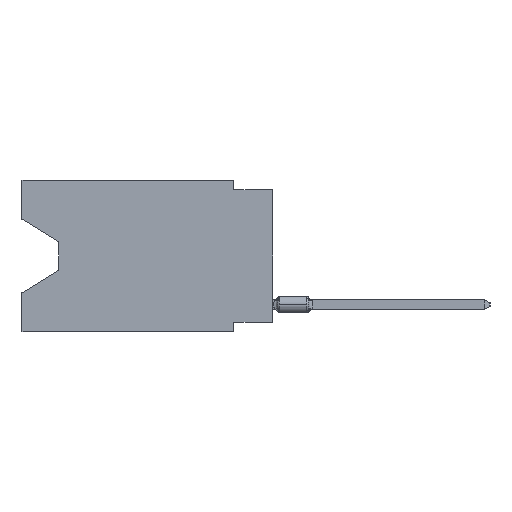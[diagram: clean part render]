
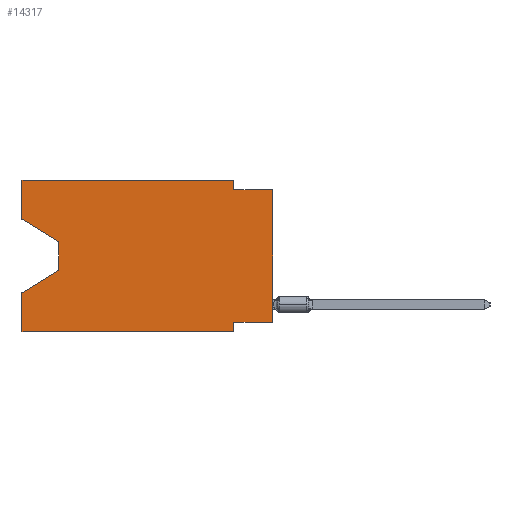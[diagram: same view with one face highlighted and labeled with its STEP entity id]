
A CAD part, left-side view. The second image highlights one B-rep face of the part: STEP entity #14317.
In plain terms, the highlighted planar face has unit normal (-1, 0, 0).
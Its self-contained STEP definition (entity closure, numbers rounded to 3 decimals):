
#158 = VERTEX_POINT ( 'NONE', #75162 ) ;
#822 = VERTEX_POINT ( 'NONE', #27262 ) ;
#1115 = FACE_OUTER_BOUND ( 'NONE', #10426, .T. ) ;
#1602 = VECTOR ( 'NONE', #66777, 1000. ) ;
#2522 = LINE ( 'NONE', #67689, #20589 ) ;
#3989 = DIRECTION ( 'NONE',  ( 0., 0., 1. ) ) ;
#4224 = ORIENTED_EDGE ( 'NONE', *, *, #29088, .T. ) ;
#4590 = CARTESIAN_POINT ( 'NONE',  ( 0., 2.54, -9.906 ) ) ;
#5325 = CARTESIAN_POINT ( 'NONE',  ( 0., 0., -0.635 ) ) ;
#5835 = VECTOR ( 'NONE', #65024, 1000. ) ;
#5856 = EDGE_CURVE ( 'NONE', #6912, #41444, #20764, .T. ) ;
#6229 = DIRECTION ( 'NONE',  ( 0., 0., -1. ) ) ;
#6878 = ORIENTED_EDGE ( 'NONE', *, *, #37665, .F. ) ;
#6912 = VERTEX_POINT ( 'NONE', #38267 ) ;
#6931 = VERTEX_POINT ( 'NONE', #55828 ) ;
#9515 = AXIS2_PLACEMENT_3D ( 'NONE', #48719, #72521, #19039 ) ;
#9548 = ORIENTED_EDGE ( 'NONE', *, *, #5856, .F. ) ;
#10426 = EDGE_LOOP ( 'NONE', ( #45156, #49991, #4224, #59094, #70288, #74477, #9548, #26184, #24464, #6878, #31904, #21497 ) ) ;
#11801 = CARTESIAN_POINT ( 'NONE',  ( 0., 2.54, -9.271 ) ) ;
#11858 = EDGE_CURVE ( 'NONE', #6931, #34887, #46647, .T. ) ;
#13762 = DIRECTION ( 'NONE',  ( 0., -1., 0. ) ) ;
#14317 = ADVANCED_FACE ( 'NONE', ( #1115 ), #24904, .F. ) ;
#14921 = DIRECTION ( 'NONE',  ( 0., 1., 0. ) ) ;
#15190 = EDGE_CURVE ( 'NONE', #44226, #27421, #27407, .T. ) ;
#15648 = LINE ( 'NONE', #68365, #43727 ) ;
#17175 = CARTESIAN_POINT ( 'NONE',  ( 0., 16.383, -7.36 ) ) ;
#17506 = VERTEX_POINT ( 'NONE', #4590 ) ;
#19039 = DIRECTION ( 'NONE',  ( 0., 0., -1. ) ) ;
#19142 = LINE ( 'NONE', #42949, #1602 ) ;
#20589 = VECTOR ( 'NONE', #73551, 1000. ) ;
#20764 = LINE ( 'NONE', #44573, #42759 ) ;
#21497 = ORIENTED_EDGE ( 'NONE', *, *, #44008, .F. ) ;
#21527 = LINE ( 'NONE', #38731, #37981 ) ;
#22171 = VERTEX_POINT ( 'NONE', #36906 ) ;
#22582 = EDGE_CURVE ( 'NONE', #822, #17506, #19142, .T. ) ;
#23460 = VECTOR ( 'NONE', #6229, 1000. ) ;
#24464 = ORIENTED_EDGE ( 'NONE', *, *, #15190, .F. ) ;
#24904 = PLANE ( 'NONE',  #9515 ) ;
#26184 = ORIENTED_EDGE ( 'NONE', *, *, #36862, .T. ) ;
#26288 = VECTOR ( 'NONE', #73059, 1000. ) ;
#26334 = CARTESIAN_POINT ( 'NONE',  ( 0., 16.383, 0. ) ) ;
#27262 = CARTESIAN_POINT ( 'NONE',  ( 0., 16.383, -9.906 ) ) ;
#27407 = LINE ( 'NONE', #44570, #45779 ) ;
#27421 = VERTEX_POINT ( 'NONE', #5325 ) ;
#27892 = LINE ( 'NONE', #51700, #48867 ) ;
#28222 = EDGE_CURVE ( 'NONE', #822, #59227, #21527, .T. ) ;
#28305 = CARTESIAN_POINT ( 'NONE',  ( 0., 16.383, -2.546 ) ) ;
#29088 = EDGE_CURVE ( 'NONE', #22171, #59227, #2522, .T. ) ;
#31703 = CARTESIAN_POINT ( 'NONE',  ( 0., 2.54, 0. ) ) ;
#31904 = ORIENTED_EDGE ( 'NONE', *, *, #43879, .F. ) ;
#34887 = VERTEX_POINT ( 'NONE', #57355 ) ;
#36335 = EDGE_CURVE ( 'NONE', #41444, #17506, #73687, .T. ) ;
#36862 = EDGE_CURVE ( 'NONE', #6912, #27421, #27892, .T. ) ;
#36906 = CARTESIAN_POINT ( 'NONE',  ( 0., 13.97, -5.893 ) ) ;
#37575 = LINE ( 'NONE', #31703, #38998 ) ;
#37665 = EDGE_CURVE ( 'NONE', #158, #44226, #37575, .T. ) ;
#37981 = VECTOR ( 'NONE', #3989, 1000. ) ;
#38267 = CARTESIAN_POINT ( 'NONE',  ( 0., 0., -9.271 ) ) ;
#38731 = CARTESIAN_POINT ( 'NONE',  ( 0., 16.383, 0. ) ) ;
#38998 = VECTOR ( 'NONE', #55138, 1000. ) ;
#39471 = DIRECTION ( 'NONE',  ( 0., 0., 1. ) ) ;
#39635 = EDGE_CURVE ( 'NONE', #34887, #22171, #43238, .T. ) ;
#41399 = CARTESIAN_POINT ( 'NONE',  ( 0., 2.54, -0.635 ) ) ;
#41444 = VERTEX_POINT ( 'NONE', #11801 ) ;
#42428 = VECTOR ( 'NONE', #49875, 1000. ) ;
#42759 = VECTOR ( 'NONE', #14921, 1000. ) ;
#42862 = CARTESIAN_POINT ( 'NONE',  ( 0., 13.97, -4.013 ) ) ;
#42949 = CARTESIAN_POINT ( 'NONE',  ( 0., 16.383, -9.906 ) ) ;
#43238 = LINE ( 'NONE', #42862, #23460 ) ;
#43727 = VECTOR ( 'NONE', #39471, 1000. ) ;
#43879 = EDGE_CURVE ( 'NONE', #66392, #158, #49639, .T. ) ;
#44008 = EDGE_CURVE ( 'NONE', #6931, #66392, #15648, .T. ) ;
#44226 = VERTEX_POINT ( 'NONE', #41399 ) ;
#44570 = CARTESIAN_POINT ( 'NONE',  ( 0., 0., -0.635 ) ) ;
#44573 = CARTESIAN_POINT ( 'NONE',  ( 0., 0., -9.271 ) ) ;
#45156 = ORIENTED_EDGE ( 'NONE', *, *, #11858, .T. ) ;
#45459 = DIRECTION ( 'NONE',  ( 0., 0., 1. ) ) ;
#45779 = VECTOR ( 'NONE', #13762, 1000. ) ;
#46647 = LINE ( 'NONE', #28305, #5835 ) ;
#48108 = CARTESIAN_POINT ( 'NONE',  ( 0., 16.383, 0. ) ) ;
#48719 = CARTESIAN_POINT ( 'NONE',  ( 0., 16.383, 0. ) ) ;
#48867 = VECTOR ( 'NONE', #45459, 1000. ) ;
#49639 = LINE ( 'NONE', #48108, #26288 ) ;
#49875 = DIRECTION ( 'NONE',  ( 0., 0., -1. ) ) ;
#49991 = ORIENTED_EDGE ( 'NONE', *, *, #39635, .T. ) ;
#51700 = CARTESIAN_POINT ( 'NONE',  ( 0., 0., 0. ) ) ;
#55138 = DIRECTION ( 'NONE',  ( 0., 0., -1. ) ) ;
#55828 = CARTESIAN_POINT ( 'NONE',  ( 0., 16.383, -2.546 ) ) ;
#57355 = CARTESIAN_POINT ( 'NONE',  ( 0., 13.97, -4.013 ) ) ;
#59094 = ORIENTED_EDGE ( 'NONE', *, *, #28222, .F. ) ;
#59227 = VERTEX_POINT ( 'NONE', #17175 ) ;
#65024 = DIRECTION ( 'NONE',  ( 0., -0.855, -0.519 ) ) ;
#66392 = VERTEX_POINT ( 'NONE', #26334 ) ;
#66681 = CARTESIAN_POINT ( 'NONE',  ( 0., 2.54, -9.906 ) ) ;
#66777 = DIRECTION ( 'NONE',  ( 0., -1., 0. ) ) ;
#67689 = CARTESIAN_POINT ( 'NONE',  ( 0., 13.97, -5.893 ) ) ;
#68365 = CARTESIAN_POINT ( 'NONE',  ( 0., 16.383, 0. ) ) ;
#70288 = ORIENTED_EDGE ( 'NONE', *, *, #22582, .T. ) ;
#72521 = DIRECTION ( 'NONE',  ( 1., 0., 0. ) ) ;
#73059 = DIRECTION ( 'NONE',  ( 0., -1., 0. ) ) ;
#73551 = DIRECTION ( 'NONE',  ( 0., 0.855, -0.519 ) ) ;
#73687 = LINE ( 'NONE', #66681, #42428 ) ;
#74477 = ORIENTED_EDGE ( 'NONE', *, *, #36335, .F. ) ;
#75162 = CARTESIAN_POINT ( 'NONE',  ( 0., 2.54, 0. ) ) ;
